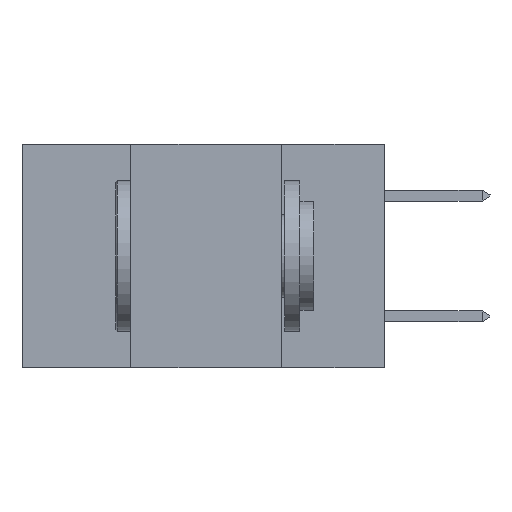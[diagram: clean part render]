
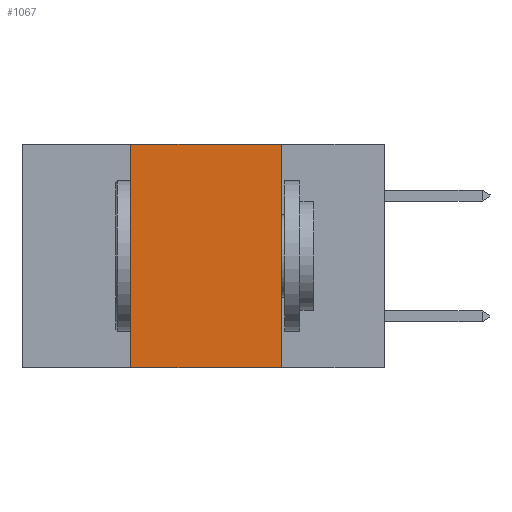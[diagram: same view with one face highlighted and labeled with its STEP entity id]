
A CAD part, left-side view. The second image highlights one B-rep face of the part: STEP entity #1067.
In plain terms, the highlighted planar face has unit normal (-1, 0, 0).
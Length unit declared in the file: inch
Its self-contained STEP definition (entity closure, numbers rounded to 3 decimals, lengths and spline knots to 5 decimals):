
#368 = EDGE_CURVE ( 'NONE', #4768, #6934, #8856, .T. ) ;
#1067 = ADVANCED_FACE ( 'NONE', ( #5068 ), #7861, .F. ) ;
#1323 = EDGE_CURVE ( 'NONE', #5371, #1361, #2235, .T. ) ;
#1361 = VERTEX_POINT ( 'NONE', #7990 ) ;
#2235 = LINE ( 'NONE', #10012, #2573 ) ;
#2357 = DIRECTION ( 'NONE',  ( 1., 0., 0. ) ) ;
#2535 = CARTESIAN_POINT ( 'NONE',  ( 0., 0.42, 0. ) ) ;
#2573 = VECTOR ( 'NONE', #9856, 39.37008 ) ;
#2673 = CARTESIAN_POINT ( 'NONE',  ( 0., 0.42, 0. ) ) ;
#2686 = ORIENTED_EDGE ( 'NONE', *, *, #1323, .F. ) ;
#3008 = CARTESIAN_POINT ( 'NONE',  ( 0., 0.6, -0.37 ) ) ;
#3611 = AXIS2_PLACEMENT_3D ( 'NONE', #11049, #2357, #8545 ) ;
#3701 = VECTOR ( 'NONE', #5566, 39.37008 ) ;
#3961 = DIRECTION ( 'NONE',  ( 0., 0., 1. ) ) ;
#4768 = VERTEX_POINT ( 'NONE', #12198 ) ;
#5068 = FACE_OUTER_BOUND ( 'NONE', #8162, .T. ) ;
#5371 = VERTEX_POINT ( 'NONE', #9970 ) ;
#5566 = DIRECTION ( 'NONE',  ( 0., -1., 0. ) ) ;
#5630 = ORIENTED_EDGE ( 'NONE', *, *, #368, .F. ) ;
#5695 = CARTESIAN_POINT ( 'NONE',  ( 0., 0.6, 0. ) ) ;
#6323 = VECTOR ( 'NONE', #3961, 39.37008 ) ;
#6560 = EDGE_CURVE ( 'NONE', #6934, #5371, #7258, .T. ) ;
#6934 = VERTEX_POINT ( 'NONE', #2673 ) ;
#7258 = LINE ( 'NONE', #5695, #3701 ) ;
#7323 = VECTOR ( 'NONE', #9702, 39.37008 ) ;
#7861 = PLANE ( 'NONE',  #3611 ) ;
#7990 = CARTESIAN_POINT ( 'NONE',  ( 0., 0.17, -0.37 ) ) ;
#8162 = EDGE_LOOP ( 'NONE', ( #2686, #10316, #5630, #8214 ) ) ;
#8214 = ORIENTED_EDGE ( 'NONE', *, *, #10755, .T. ) ;
#8545 = DIRECTION ( 'NONE',  ( 0., 0., -1. ) ) ;
#8856 = LINE ( 'NONE', #2535, #6323 ) ;
#9702 = DIRECTION ( 'NONE',  ( 0., -1., 0. ) ) ;
#9754 = LINE ( 'NONE', #3008, #7323 ) ;
#9856 = DIRECTION ( 'NONE',  ( 0., 0., -1. ) ) ;
#9970 = CARTESIAN_POINT ( 'NONE',  ( 0., 0.17, 0. ) ) ;
#10012 = CARTESIAN_POINT ( 'NONE',  ( 0., 0.17, 0. ) ) ;
#10316 = ORIENTED_EDGE ( 'NONE', *, *, #6560, .F. ) ;
#10755 = EDGE_CURVE ( 'NONE', #4768, #1361, #9754, .T. ) ;
#11049 = CARTESIAN_POINT ( 'NONE',  ( 0., 0.6, 0. ) ) ;
#12198 = CARTESIAN_POINT ( 'NONE',  ( 0., 0.42, -0.37 ) ) ;
